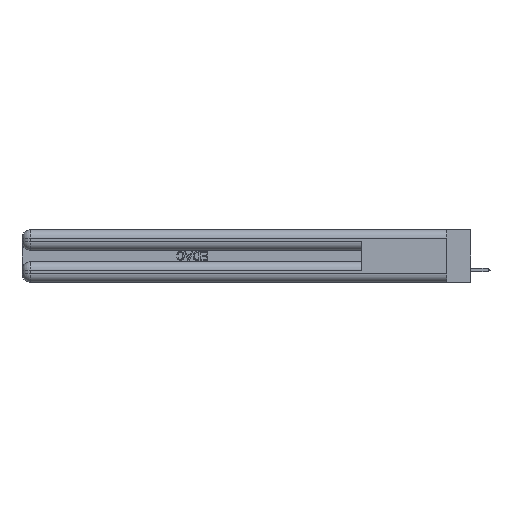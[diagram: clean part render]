
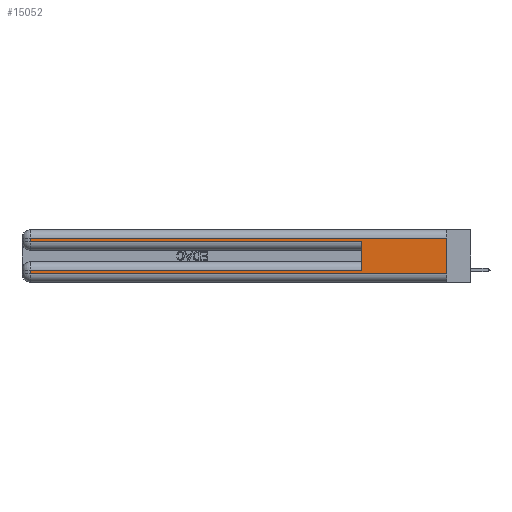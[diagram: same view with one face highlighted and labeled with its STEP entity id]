
A CAD part, left-side view. The second image highlights one B-rep face of the part: STEP entity #15052.
In plain terms, the highlighted planar face has unit normal (-1, 0, 0).
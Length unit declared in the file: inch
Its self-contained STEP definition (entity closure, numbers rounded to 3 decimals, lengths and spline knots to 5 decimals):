
#24 = AXIS2_PLACEMENT_3D ( 'NONE', #22151, #31182, #25141 ) ;
#130 = VECTOR ( 'NONE', #17458, 39.37008 ) ;
#2738 = VERTEX_POINT ( 'NONE', #7365 ) ;
#3080 = VECTOR ( 'NONE', #10096, 39.37008 ) ;
#3843 = VECTOR ( 'NONE', #27024, 39.37008 ) ;
#3915 = ORIENTED_EDGE ( 'NONE', *, *, #5216, .F. ) ;
#3987 = VECTOR ( 'NONE', #30053, 39.37008 ) ;
#5216 = EDGE_CURVE ( 'NONE', #9164, #36919, #8063, .T. ) ;
#6007 = EDGE_CURVE ( 'NONE', #9164, #25574, #29434, .T. ) ;
#6572 = EDGE_CURVE ( 'NONE', #26667, #32911, #37602, .T. ) ;
#7365 = CARTESIAN_POINT ( 'NONE',  ( 0., 0.6, 0.085 ) ) ;
#8063 = LINE ( 'NONE', #17336, #130 ) ;
#9164 = VERTEX_POINT ( 'NONE', #25716 ) ;
#9411 = CARTESIAN_POINT ( 'NONE',  ( 0., 0., 0.285 ) ) ;
#9489 = DIRECTION ( 'NONE',  ( 0., 1., 0. ) ) ;
#10096 = DIRECTION ( 'NONE',  ( 0., 0., 1. ) ) ;
#10493 = LINE ( 'NONE', #13483, #3080 ) ;
#12064 = EDGE_CURVE ( 'NONE', #2738, #32911, #10493, .T. ) ;
#12360 = ORIENTED_EDGE ( 'NONE', *, *, #6007, .T. ) ;
#12371 = VECTOR ( 'NONE', #38034, 39.37008 ) ;
#12377 = CARTESIAN_POINT ( 'NONE',  ( 0., 2.94, 0.06 ) ) ;
#13121 = LINE ( 'NONE', #24064, #3843 ) ;
#13483 = CARTESIAN_POINT ( 'NONE',  ( 0., 0.6, 0.145 ) ) ;
#15052 = ADVANCED_FACE ( 'NONE', ( #33275 ), #27974, .F. ) ;
#15926 = CARTESIAN_POINT ( 'NONE',  ( 0., 0.6, 0.285 ) ) ;
#17336 = CARTESIAN_POINT ( 'NONE',  ( 0., 0., 0.37 ) ) ;
#17458 = DIRECTION ( 'NONE',  ( 0., 0., -1. ) ) ;
#17849 = VERTEX_POINT ( 'NONE', #12377 ) ;
#19470 = LINE ( 'NONE', #35101, #22762 ) ;
#19758 = EDGE_CURVE ( 'NONE', #25574, #26667, #13121, .T. ) ;
#21330 = EDGE_CURVE ( 'NONE', #2738, #29161, #19470, .T. ) ;
#22151 = CARTESIAN_POINT ( 'NONE',  ( 0., 0., 0.37 ) ) ;
#22293 = DIRECTION ( 'NONE',  ( 0., -1., 0. ) ) ;
#22493 = LINE ( 'NONE', #30382, #29384 ) ;
#22762 = VECTOR ( 'NONE', #32530, 39.37008 ) ;
#23166 = ORIENTED_EDGE ( 'NONE', *, *, #29214, .T. ) ;
#23582 = ORIENTED_EDGE ( 'NONE', *, *, #6572, .T. ) ;
#23664 = ORIENTED_EDGE ( 'NONE', *, *, #19758, .T. ) ;
#24064 = CARTESIAN_POINT ( 'NONE',  ( 0., 2.94, 0.37 ) ) ;
#25141 = DIRECTION ( 'NONE',  ( 0., 0., -1. ) ) ;
#25574 = VERTEX_POINT ( 'NONE', #36757 ) ;
#25716 = CARTESIAN_POINT ( 'NONE',  ( 0., 0., 0.31 ) ) ;
#26464 = ORIENTED_EDGE ( 'NONE', *, *, #21330, .T. ) ;
#26667 = VERTEX_POINT ( 'NONE', #36622 ) ;
#27015 = CARTESIAN_POINT ( 'NONE',  ( 0., 0., 0.06 ) ) ;
#27024 = DIRECTION ( 'NONE',  ( 0., 0., -1. ) ) ;
#27974 = PLANE ( 'NONE',  #24 ) ;
#29161 = VERTEX_POINT ( 'NONE', #29240 ) ;
#29214 = EDGE_CURVE ( 'NONE', #29161, #17849, #33110, .T. ) ;
#29240 = CARTESIAN_POINT ( 'NONE',  ( 0., 2.94, 0.085 ) ) ;
#29384 = VECTOR ( 'NONE', #22293, 39.37008 ) ;
#29434 = LINE ( 'NONE', #38086, #30840 ) ;
#30053 = DIRECTION ( 'NONE',  ( 0., -1., 0. ) ) ;
#30382 = CARTESIAN_POINT ( 'NONE',  ( 0., 0., 0.06 ) ) ;
#30840 = VECTOR ( 'NONE', #9489, 39.37008 ) ;
#30927 = ORIENTED_EDGE ( 'NONE', *, *, #30985, .T. ) ;
#30985 = EDGE_CURVE ( 'NONE', #17849, #36919, #22493, .T. ) ;
#31182 = DIRECTION ( 'NONE',  ( 1., 0., 0. ) ) ;
#32201 = CARTESIAN_POINT ( 'NONE',  ( 0., 2.94, 0.37 ) ) ;
#32530 = DIRECTION ( 'NONE',  ( 0., 1., 0. ) ) ;
#32911 = VERTEX_POINT ( 'NONE', #15926 ) ;
#33110 = LINE ( 'NONE', #32201, #12371 ) ;
#33275 = FACE_OUTER_BOUND ( 'NONE', #35603, .T. ) ;
#35101 = CARTESIAN_POINT ( 'NONE',  ( 0., 0., 0.085 ) ) ;
#35603 = EDGE_LOOP ( 'NONE', ( #3915, #12360, #23664, #23582, #35745, #26464, #23166, #30927 ) ) ;
#35745 = ORIENTED_EDGE ( 'NONE', *, *, #12064, .F. ) ;
#36622 = CARTESIAN_POINT ( 'NONE',  ( 0., 2.94, 0.285 ) ) ;
#36757 = CARTESIAN_POINT ( 'NONE',  ( 0., 2.94, 0.31 ) ) ;
#36919 = VERTEX_POINT ( 'NONE', #27015 ) ;
#37602 = LINE ( 'NONE', #9411, #3987 ) ;
#38034 = DIRECTION ( 'NONE',  ( 0., 0., -1. ) ) ;
#38086 = CARTESIAN_POINT ( 'NONE',  ( 0., 0., 0.31 ) ) ;
